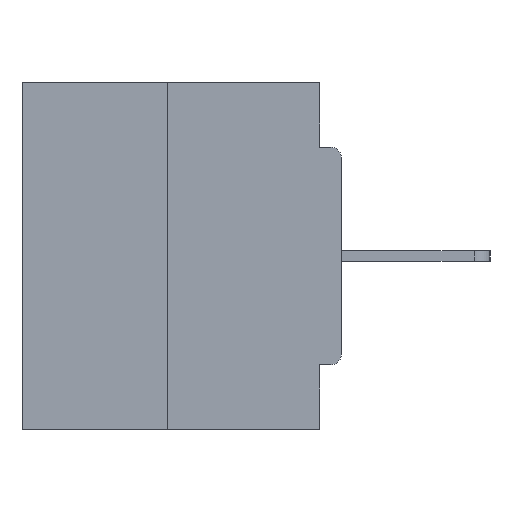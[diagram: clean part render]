
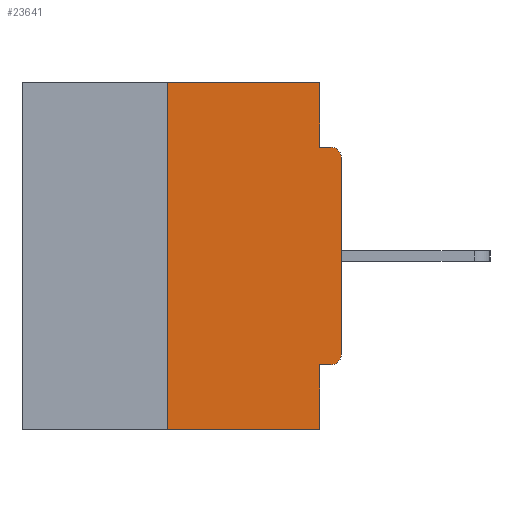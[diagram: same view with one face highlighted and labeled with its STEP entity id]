
A CAD part, left-side view. The second image highlights one B-rep face of the part: STEP entity #23641.
In plain terms, the highlighted planar face has unit normal (-1, 0, 0).
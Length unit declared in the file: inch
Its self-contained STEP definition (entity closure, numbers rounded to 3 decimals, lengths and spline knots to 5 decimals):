
#14 = DIRECTION ( 'NONE',  ( 0., 0., -1. ) ) ;
#105 = CARTESIAN_POINT ( 'NONE',  ( 0., 0.031, 0. ) ) ;
#724 = EDGE_CURVE ( 'NONE', #10637, #21759, #7210, .T. ) ;
#1589 = EDGE_CURVE ( 'NONE', #5072, #11322, #9004, .T. ) ;
#2268 = VERTEX_POINT ( 'NONE', #9405 ) ;
#2606 = DIRECTION ( 'NONE',  ( -1., 0., 0. ) ) ;
#2805 = VERTEX_POINT ( 'NONE', #30659 ) ;
#3794 = DIRECTION ( 'NONE',  ( 0., -1., 0. ) ) ;
#4309 = EDGE_CURVE ( 'NONE', #2805, #6254, #27355, .T. ) ;
#4930 = DIRECTION ( 'NONE',  ( 1., 0., 0. ) ) ;
#5072 = VERTEX_POINT ( 'NONE', #24269 ) ;
#5621 = ORIENTED_EDGE ( 'NONE', *, *, #14731, .T. ) ;
#6152 = EDGE_CURVE ( 'NONE', #6254, #14271, #13260, .T. ) ;
#6254 = VERTEX_POINT ( 'NONE', #8822 ) ;
#6596 = DIRECTION ( 'NONE',  ( 0., -1., 0. ) ) ;
#6772 = VECTOR ( 'NONE', #22831, 39.37008 ) ;
#6850 = ORIENTED_EDGE ( 'NONE', *, *, #22777, .T. ) ;
#7210 = LINE ( 'NONE', #14890, #6772 ) ;
#7915 = EDGE_CURVE ( 'NONE', #21759, #10818, #32638, .T. ) ;
#8822 = CARTESIAN_POINT ( 'NONE',  ( 0., 0.031, 0. ) ) ;
#9004 = CIRCLE ( 'NONE', #22724, 0.015 ) ;
#9138 = CARTESIAN_POINT ( 'NONE',  ( 0., 0.031, -0.5 ) ) ;
#9405 = CARTESIAN_POINT ( 'NONE',  ( 0., 0.25, -0.5 ) ) ;
#9712 = AXIS2_PLACEMENT_3D ( 'NONE', #12505, #2606, #14 ) ;
#9715 = CARTESIAN_POINT ( 'NONE',  ( 0., 0.46, 0. ) ) ;
#10158 = CARTESIAN_POINT ( 'NONE',  ( 0., 0.46, -0.5 ) ) ;
#10464 = LINE ( 'NONE', #29354, #19748 ) ;
#10637 = VERTEX_POINT ( 'NONE', #27159 ) ;
#10818 = VERTEX_POINT ( 'NONE', #17642 ) ;
#10983 = ORIENTED_EDGE ( 'NONE', *, *, #21168, .T. ) ;
#11322 = VERTEX_POINT ( 'NONE', #20859 ) ;
#11549 = CARTESIAN_POINT ( 'NONE',  ( 0., 0.46, 0. ) ) ;
#12505 = CARTESIAN_POINT ( 'NONE',  ( 0., 0.015, -0.3915 ) ) ;
#12871 = DIRECTION ( 'NONE',  ( 0., -1., 0. ) ) ;
#12996 = CARTESIAN_POINT ( 'NONE',  ( 0., 0.031, -0.4065 ) ) ;
#13199 = DIRECTION ( 'NONE',  ( 0., 0., -1. ) ) ;
#13260 = LINE ( 'NONE', #105, #26030 ) ;
#14271 = VERTEX_POINT ( 'NONE', #25806 ) ;
#14648 = AXIS2_PLACEMENT_3D ( 'NONE', #9715, #4930, #30841 ) ;
#14731 = EDGE_CURVE ( 'NONE', #30921, #5072, #31716, .T. ) ;
#14890 = CARTESIAN_POINT ( 'NONE',  ( 0., 0., -0.4065 ) ) ;
#14951 = ORIENTED_EDGE ( 'NONE', *, *, #724, .F. ) ;
#15684 = CIRCLE ( 'NONE', #9712, 0.015 ) ;
#15762 = DIRECTION ( 'NONE',  ( -1., 0., 0. ) ) ;
#15886 = DIRECTION ( 'NONE',  ( 0., 0., 1. ) ) ;
#16076 = VECTOR ( 'NONE', #6596, 39.37008 ) ;
#16153 = ORIENTED_EDGE ( 'NONE', *, *, #6152, .F. ) ;
#17642 = CARTESIAN_POINT ( 'NONE',  ( 0., 0.031, -0.5 ) ) ;
#18378 = ORIENTED_EDGE ( 'NONE', *, *, #4309, .F. ) ;
#19748 = VECTOR ( 'NONE', #3794, 39.37008 ) ;
#20186 = CARTESIAN_POINT ( 'NONE',  ( 0., 0.25, 0. ) ) ;
#20859 = CARTESIAN_POINT ( 'NONE',  ( 0., 0.015, -0.0935 ) ) ;
#21168 = EDGE_CURVE ( 'NONE', #2268, #10818, #33516, .T. ) ;
#21409 = CARTESIAN_POINT ( 'NONE',  ( 0., 0., 0. ) ) ;
#21664 = DIRECTION ( 'NONE',  ( 0., 0., -1. ) ) ;
#21759 = VERTEX_POINT ( 'NONE', #12996 ) ;
#22724 = AXIS2_PLACEMENT_3D ( 'NONE', #31114, #15762, #13199 ) ;
#22777 = EDGE_CURVE ( 'NONE', #10637, #30921, #15684, .T. ) ;
#22831 = DIRECTION ( 'NONE',  ( 0., 1., 0. ) ) ;
#22933 = FACE_OUTER_BOUND ( 'NONE', #30019, .T. ) ;
#23641 = ADVANCED_FACE ( 'NONE', ( #22933 ), #31010, .F. ) ;
#23945 = ORIENTED_EDGE ( 'NONE', *, *, #7915, .F. ) ;
#24059 = CARTESIAN_POINT ( 'NONE',  ( 0., 0., -0.3915 ) ) ;
#24269 = CARTESIAN_POINT ( 'NONE',  ( 0., 0., -0.1085 ) ) ;
#25806 = CARTESIAN_POINT ( 'NONE',  ( 0., 0.031, -0.0935 ) ) ;
#26030 = VECTOR ( 'NONE', #33880, 39.37008 ) ;
#26299 = VECTOR ( 'NONE', #15886, 39.37008 ) ;
#27159 = CARTESIAN_POINT ( 'NONE',  ( 0., 0.015, -0.4065 ) ) ;
#27353 = ORIENTED_EDGE ( 'NONE', *, *, #27457, .F. ) ;
#27355 = LINE ( 'NONE', #11549, #16076 ) ;
#27457 = EDGE_CURVE ( 'NONE', #14271, #11322, #10464, .T. ) ;
#27809 = VECTOR ( 'NONE', #12871, 39.37008 ) ;
#28129 = EDGE_CURVE ( 'NONE', #2268, #2805, #29996, .T. ) ;
#28575 = VECTOR ( 'NONE', #30356, 39.37008 ) ;
#29354 = CARTESIAN_POINT ( 'NONE',  ( 0., 0., -0.0935 ) ) ;
#29996 = LINE ( 'NONE', #20186, #28575 ) ;
#30019 = EDGE_LOOP ( 'NONE', ( #18378, #32308, #10983, #23945, #14951, #6850, #5621, #32910, #27353, #16153 ) ) ;
#30356 = DIRECTION ( 'NONE',  ( 0., 0., 1. ) ) ;
#30659 = CARTESIAN_POINT ( 'NONE',  ( 0., 0.25, 0. ) ) ;
#30841 = DIRECTION ( 'NONE',  ( 0., 0., -1. ) ) ;
#30921 = VERTEX_POINT ( 'NONE', #24059 ) ;
#31010 = PLANE ( 'NONE',  #14648 ) ;
#31114 = CARTESIAN_POINT ( 'NONE',  ( 0., 0.015, -0.1085 ) ) ;
#31123 = VECTOR ( 'NONE', #21664, 39.37008 ) ;
#31716 = LINE ( 'NONE', #21409, #26299 ) ;
#32308 = ORIENTED_EDGE ( 'NONE', *, *, #28129, .F. ) ;
#32638 = LINE ( 'NONE', #9138, #31123 ) ;
#32910 = ORIENTED_EDGE ( 'NONE', *, *, #1589, .T. ) ;
#33516 = LINE ( 'NONE', #10158, #27809 ) ;
#33880 = DIRECTION ( 'NONE',  ( 0., 0., -1. ) ) ;
